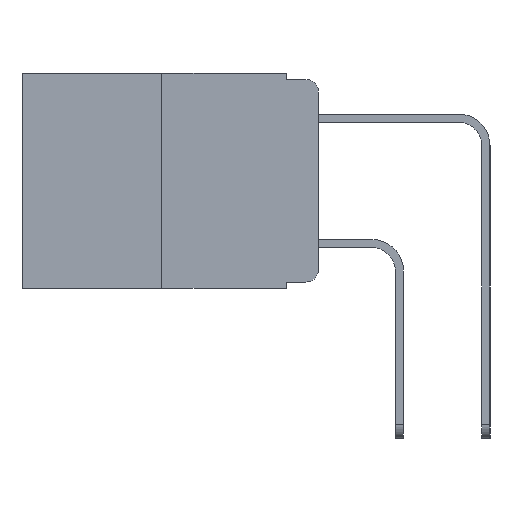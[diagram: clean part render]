
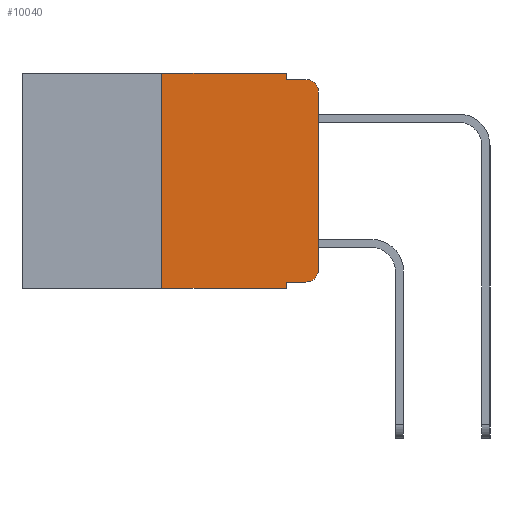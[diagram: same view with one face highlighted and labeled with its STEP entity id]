
A CAD part, left-side view. The second image highlights one B-rep face of the part: STEP entity #10040.
In plain terms, the highlighted planar face has unit normal (-1, 0, 0).
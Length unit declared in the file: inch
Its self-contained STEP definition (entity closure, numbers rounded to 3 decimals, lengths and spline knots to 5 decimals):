
#10 = LINE ( 'NONE', #3073, #12300 ) ;
#18 = VERTEX_POINT ( 'NONE', #4678 ) ;
#37 = AXIS2_PLACEMENT_3D ( 'NONE', #2585, #9550, #3651 ) ;
#53 = ORIENTED_EDGE ( 'NONE', *, *, #2303, .F. ) ;
#221 = FACE_OUTER_BOUND ( 'NONE', #9958, .T. ) ;
#435 = EDGE_CURVE ( 'NONE', #5107, #5868, #823, .T. ) ;
#586 = CARTESIAN_POINT ( 'NONE',  ( 0., 0., -0.313 ) ) ;
#615 = CARTESIAN_POINT ( 'NONE',  ( 0., 0.473, -0.343 ) ) ;
#823 = LINE ( 'NONE', #4574, #5941 ) ;
#853 = VERTEX_POINT ( 'NONE', #12778 ) ;
#909 = DIRECTION ( 'NONE',  ( 0., -1., 0. ) ) ;
#1180 = CARTESIAN_POINT ( 'NONE',  ( 0., 0.25, -0.343 ) ) ;
#1259 = LINE ( 'NONE', #615, #9007 ) ;
#1303 = VECTOR ( 'NONE', #11984, 39.37008 ) ;
#1359 = VERTEX_POINT ( 'NONE', #12524 ) ;
#1462 = EDGE_CURVE ( 'NONE', #9587, #2668, #12700, .T. ) ;
#1571 = CARTESIAN_POINT ( 'NONE',  ( 0., 0.02, -0.333 ) ) ;
#2040 = DIRECTION ( 'NONE',  ( 0., -1., 0. ) ) ;
#2303 = EDGE_CURVE ( 'NONE', #5868, #18, #3951, .T. ) ;
#2404 = ORIENTED_EDGE ( 'NONE', *, *, #12739, .F. ) ;
#2585 = CARTESIAN_POINT ( 'NONE',  ( 0., 0.02, -0.313 ) ) ;
#2590 = CARTESIAN_POINT ( 'NONE',  ( 0., 0.051, -0.343 ) ) ;
#2626 = ORIENTED_EDGE ( 'NONE', *, *, #8146, .F. ) ;
#2659 = VECTOR ( 'NONE', #909, 39.37008 ) ;
#2668 = VERTEX_POINT ( 'NONE', #1571 ) ;
#2706 = CARTESIAN_POINT ( 'NONE',  ( 0., 0., 0. ) ) ;
#2791 = CARTESIAN_POINT ( 'NONE',  ( 0., 0.02, -0.03 ) ) ;
#2793 = EDGE_CURVE ( 'NONE', #7039, #3402, #1259, .T. ) ;
#3001 = LINE ( 'NONE', #2706, #7939 ) ;
#3073 = CARTESIAN_POINT ( 'NONE',  ( 0., 0.051, 0. ) ) ;
#3402 = VERTEX_POINT ( 'NONE', #2590 ) ;
#3425 = CIRCLE ( 'NONE', #5300, 0.02 ) ;
#3651 = DIRECTION ( 'NONE',  ( 0., 0., -1. ) ) ;
#3688 = DIRECTION ( 'NONE',  ( 0., 0., -1. ) ) ;
#3762 = DIRECTION ( 'NONE',  ( 0., 0., 1. ) ) ;
#3789 = EDGE_CURVE ( 'NONE', #1359, #18, #3425, .T. ) ;
#3951 = LINE ( 'NONE', #5020, #11387 ) ;
#4241 = CARTESIAN_POINT ( 'NONE',  ( 0., 0.25, 0. ) ) ;
#4313 = ORIENTED_EDGE ( 'NONE', *, *, #8473, .T. ) ;
#4574 = CARTESIAN_POINT ( 'NONE',  ( 0., 0.051, 0. ) ) ;
#4598 = PLANE ( 'NONE',  #4953 ) ;
#4678 = CARTESIAN_POINT ( 'NONE',  ( 0., 0.02, -0.01 ) ) ;
#4953 = AXIS2_PLACEMENT_3D ( 'NONE', #6570, #9590, #3688 ) ;
#4955 = CARTESIAN_POINT ( 'NONE',  ( 0., 0.051, -0.01 ) ) ;
#5020 = CARTESIAN_POINT ( 'NONE',  ( 0., 0.051, -0.01 ) ) ;
#5074 = DIRECTION ( 'NONE',  ( 0., 0., -1. ) ) ;
#5107 = VERTEX_POINT ( 'NONE', #9496 ) ;
#5280 = DIRECTION ( 'NONE',  ( 0., 0., -1. ) ) ;
#5300 = AXIS2_PLACEMENT_3D ( 'NONE', #2791, #8690, #6847 ) ;
#5399 = VECTOR ( 'NONE', #12161, 39.37008 ) ;
#5588 = ORIENTED_EDGE ( 'NONE', *, *, #3789, .T. ) ;
#5741 = VERTEX_POINT ( 'NONE', #586 ) ;
#5868 = VERTEX_POINT ( 'NONE', #4955 ) ;
#5937 = ORIENTED_EDGE ( 'NONE', *, *, #7734, .T. ) ;
#5941 = VECTOR ( 'NONE', #5280, 39.37008 ) ;
#6570 = CARTESIAN_POINT ( 'NONE',  ( 0., 0.473, 0. ) ) ;
#6847 = DIRECTION ( 'NONE',  ( 0., 0., -1. ) ) ;
#7039 = VERTEX_POINT ( 'NONE', #1180 ) ;
#7292 = ORIENTED_EDGE ( 'NONE', *, *, #11514, .F. ) ;
#7734 = EDGE_CURVE ( 'NONE', #2668, #5741, #11558, .T. ) ;
#7939 = VECTOR ( 'NONE', #3762, 39.37008 ) ;
#8146 = EDGE_CURVE ( 'NONE', #7039, #853, #11848, .T. ) ;
#8345 = CARTESIAN_POINT ( 'NONE',  ( 0., 0.473, 0. ) ) ;
#8473 = EDGE_CURVE ( 'NONE', #5741, #1359, #3001, .T. ) ;
#8690 = DIRECTION ( 'NONE',  ( -1., 0., 0. ) ) ;
#8903 = ORIENTED_EDGE ( 'NONE', *, *, #1462, .T. ) ;
#8974 = DIRECTION ( 'NONE',  ( 0., -1., 0. ) ) ;
#9007 = VECTOR ( 'NONE', #8974, 39.37008 ) ;
#9010 = CARTESIAN_POINT ( 'NONE',  ( 0., 0.051, -0.333 ) ) ;
#9496 = CARTESIAN_POINT ( 'NONE',  ( 0., 0.051, 0. ) ) ;
#9550 = DIRECTION ( 'NONE',  ( -1., 0., 0. ) ) ;
#9587 = VERTEX_POINT ( 'NONE', #10751 ) ;
#9590 = DIRECTION ( 'NONE',  ( 1., 0., 0. ) ) ;
#9601 = ORIENTED_EDGE ( 'NONE', *, *, #435, .F. ) ;
#9958 = EDGE_LOOP ( 'NONE', ( #4313, #5588, #53, #9601, #2404, #2626, #12113, #7292, #8903, #5937 ) ) ;
#10040 = ADVANCED_FACE ( 'NONE', ( #221 ), #4598, .F. ) ;
#10080 = LINE ( 'NONE', #8345, #5399 ) ;
#10751 = CARTESIAN_POINT ( 'NONE',  ( 0., 0.051, -0.333 ) ) ;
#11387 = VECTOR ( 'NONE', #2040, 39.37008 ) ;
#11514 = EDGE_CURVE ( 'NONE', #9587, #3402, #10, .T. ) ;
#11558 = CIRCLE ( 'NONE', #37, 0.02 ) ;
#11848 = LINE ( 'NONE', #4241, #1303 ) ;
#11984 = DIRECTION ( 'NONE',  ( 0., 0., 1. ) ) ;
#12113 = ORIENTED_EDGE ( 'NONE', *, *, #2793, .T. ) ;
#12161 = DIRECTION ( 'NONE',  ( 0., -1., 0. ) ) ;
#12300 = VECTOR ( 'NONE', #5074, 39.37008 ) ;
#12524 = CARTESIAN_POINT ( 'NONE',  ( 0., 0., -0.03 ) ) ;
#12700 = LINE ( 'NONE', #9010, #2659 ) ;
#12739 = EDGE_CURVE ( 'NONE', #853, #5107, #10080, .T. ) ;
#12778 = CARTESIAN_POINT ( 'NONE',  ( 0., 0.25, 0. ) ) ;
